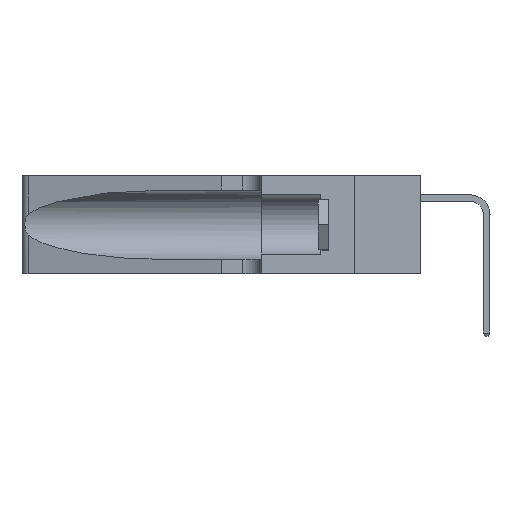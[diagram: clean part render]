
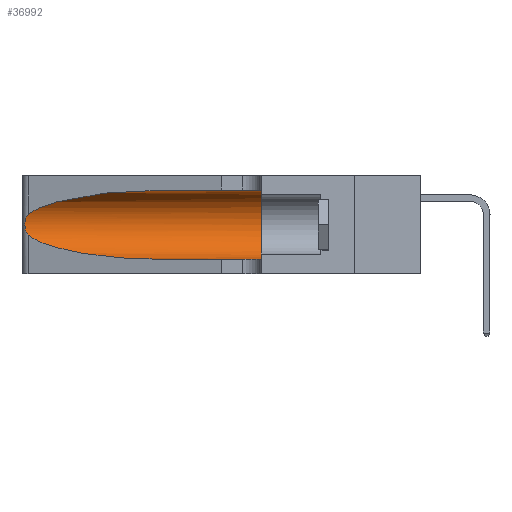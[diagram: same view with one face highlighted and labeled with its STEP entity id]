
A CAD part, left-side view. The second image highlights one B-rep face of the part: STEP entity #36992.
In plain terms, the highlighted cylindrical face has radius 3.308 mm (diameter 6.617 mm), a partial arc.
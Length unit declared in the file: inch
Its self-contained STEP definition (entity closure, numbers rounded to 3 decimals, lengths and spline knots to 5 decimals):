
#2762 = CARTESIAN_POINT ( 'NONE',  ( 0.26018, 1.23835, 0.19895 ) ) ;
#4239 = VECTOR ( 'NONE', #39506, 39.37008 ) ;
#4840 = CARTESIAN_POINT ( 'NONE',  ( 0.1305, 1.61858, 0.05475 ) ) ;
#5601 = CARTESIAN_POINT ( 'NONE',  ( 0.25487, 1.22718, 0.14631 ) ) ;
#6692 = CARTESIAN_POINT ( 'NONE',  ( 0.26075, 1.23896, 0.178 ) ) ;
#6859 = FACE_OUTER_BOUND ( 'NONE', #25412, .T. ) ;
#7450 = CARTESIAN_POINT ( 'NONE',  ( 0.2373, 1.15595, 0.08982 ) ) ;
#9319 = DIRECTION ( 'NONE',  ( 0., -1., 0. ) ) ;
#9712 = CARTESIAN_POINT ( 'NONE',  ( 0.25487, 1.22718, 0.22369 ) ) ;
#10276 = EDGE_CURVE ( 'NONE', #11919, #13698, #40772, .T. ) ;
#10569 = CARTESIAN_POINT ( 'NONE',  ( 0.25856, 1.23593, 0.16098 ) ) ;
#11341 = CARTESIAN_POINT ( 'NONE',  ( 0.1305, 0.35, 0.185 ) ) ;
#11919 = VERTEX_POINT ( 'NONE', #27972 ) ;
#12589 = ORIENTED_EDGE ( 'NONE', *, *, #13298, .T. ) ;
#12993 = CARTESIAN_POINT ( 'NONE',  ( 0.1305, 1.61858, 0.185 ) ) ;
#13034 = CARTESIAN_POINT ( 'NONE',  ( 0.1305, 1.61858, 0.31525 ) ) ;
#13298 = EDGE_CURVE ( 'NONE', #17038, #47004, #18634, .T. ) ;
#13664 = EDGE_CURVE ( 'NONE', #35030, #39182, #22699, .T. ) ;
#13698 = VERTEX_POINT ( 'NONE', #15525 ) ;
#14442 = ORIENTED_EDGE ( 'NONE', *, *, #18307, .T. ) ;
#14448 = CARTESIAN_POINT ( 'NONE',  ( 0.25639, 1.23186, 0.15144 ) ) ;
#15202 = CARTESIAN_POINT ( 'NONE',  ( 0.25487, 1.22718, 0.14631 ) ) ;
#15211 = DIRECTION ( 'NONE',  ( 0., 0., 1. ) ) ;
#15525 = CARTESIAN_POINT ( 'NONE',  ( 0.1305, 0.35, 0.05475 ) ) ;
#16726 = CARTESIAN_POINT ( 'NONE',  ( 0.2373, 1.15595, 0.28018 ) ) ;
#17038 = VERTEX_POINT ( 'NONE', #23335 ) ;
#18133 = CARTESIAN_POINT ( 'NONE',  ( 0.25487, 1.22718, 0.22369 ) ) ;
#18303 = CARTESIAN_POINT ( 'NONE',  ( 0.25487, 1.22718, 0.14631 ) ) ;
#18307 = EDGE_CURVE ( 'NONE', #39182, #13698, #36179, .T. ) ;
#18634 =( BOUNDED_CURVE ( )  B_SPLINE_CURVE ( 3, ( #47461, #20584, #16726, #24452 ),
 .UNSPECIFIED., .F., .F. ) 
 B_SPLINE_CURVE_WITH_KNOTS ( ( 4, 4 ),
 ( 1.5708, 2.84003 ),
 .UNSPECIFIED. ) 
 CURVE ( )  GEOMETRIC_REPRESENTATION_ITEM ( )  RATIONAL_B_SPLINE_CURVE ( ( 1., 0.87, 0.87, 1. ) ) 
 REPRESENTATION_ITEM ( '' )  );
#20584 = CARTESIAN_POINT ( 'NONE',  ( 0.18966, 0.96281, 0.31525 ) ) ;
#20757 = AXIS2_PLACEMENT_3D ( 'NONE', #11341, #38213, #15211 ) ;
#21016 = ORIENTED_EDGE ( 'NONE', *, *, #13664, .T. ) ;
#21658 = VECTOR ( 'NONE', #9319, 39.37008 ) ;
#22022 = CARTESIAN_POINT ( 'NONE',  ( 0.25639, 1.23184, 0.21858 ) ) ;
#22699 =( BOUNDED_CURVE ( )  B_SPLINE_CURVE ( 3, ( #15202, #7450, #49630, #42070 ),
 .UNSPECIFIED., .F., .F. ) 
 B_SPLINE_CURVE_WITH_KNOTS ( ( 4, 4 ),
 ( 3.44316, 4.71239 ),
 .UNSPECIFIED. ) 
 CURVE ( )  GEOMETRIC_REPRESENTATION_ITEM ( )  RATIONAL_B_SPLINE_CURVE ( ( 1., 0.87, 0.87, 1. ) ) 
 REPRESENTATION_ITEM ( '' )  );
#22843 = ORIENTED_EDGE ( 'NONE', *, *, #26994, .T. ) ;
#23335 = CARTESIAN_POINT ( 'NONE',  ( 0.1305, 0.72297, 0.31525 ) ) ;
#23591 = AXIS2_PLACEMENT_3D ( 'NONE', #12993, #47426, #39866 ) ;
#24452 = CARTESIAN_POINT ( 'NONE',  ( 0.25487, 1.22718, 0.22369 ) ) ;
#25412 = EDGE_LOOP ( 'NONE', ( #12589, #22843, #21016, #14442, #38484, #48712 ) ) ;
#25880 = CARTESIAN_POINT ( 'NONE',  ( 0.25854, 1.2359, 0.20912 ) ) ;
#26994 = EDGE_CURVE ( 'NONE', #47004, #35030, #39233, .T. ) ;
#27972 = CARTESIAN_POINT ( 'NONE',  ( 0.1305, 0.35, 0.31525 ) ) ;
#29728 = CARTESIAN_POINT ( 'NONE',  ( 0.26075, 1.23896, 0.19203 ) ) ;
#33606 = CARTESIAN_POINT ( 'NONE',  ( 0.26017, 1.23833, 0.17102 ) ) ;
#35030 = VERTEX_POINT ( 'NONE', #5601 ) ;
#35512 = LINE ( 'NONE', #13034, #21658 ) ;
#36179 = LINE ( 'NONE', #4840, #4239 ) ;
#36338 = CYLINDRICAL_SURFACE ( 'NONE', #23591, 0.13025 ) ;
#36992 = ADVANCED_FACE ( 'NONE', ( #6859 ), #36338, .F. ) ;
#37299 = CARTESIAN_POINT ( 'NONE',  ( 0.25555, 1.22994, 0.2215 ) ) ;
#37469 = CARTESIAN_POINT ( 'NONE',  ( 0.25789, 1.23486, 0.15765 ) ) ;
#38213 = DIRECTION ( 'NONE',  ( 0., 1., 0. ) ) ;
#38484 = ORIENTED_EDGE ( 'NONE', *, *, #10276, .F. ) ;
#39182 = VERTEX_POINT ( 'NONE', #48930 ) ;
#39233 = B_SPLINE_CURVE_WITH_KNOTS ( 'NONE', 3,
 ( #18133, #37299, #22022, #48893, #25880, #2762, #29728, #6692, #33606, #10569, #37469, #14448, #41334, #18303 ),
 .UNSPECIFIED., .F., .F.,
 ( 4, 2, 2, 2, 2, 2, 4 ),
 ( 0., 0.00027, 0.00053, 0.00107, 0.0016, 0.00187, 0.00214 ),
 .UNSPECIFIED. ) ;
#39506 = DIRECTION ( 'NONE',  ( 0., -1., 0. ) ) ;
#39866 = DIRECTION ( 'NONE',  ( 0., 0., -1. ) ) ;
#40772 = CIRCLE ( 'NONE', #20757, 0.13025 ) ;
#41334 = CARTESIAN_POINT ( 'NONE',  ( 0.25555, 1.22993, 0.14849 ) ) ;
#42070 = CARTESIAN_POINT ( 'NONE',  ( 0.1305, 0.72297, 0.05475 ) ) ;
#47004 = VERTEX_POINT ( 'NONE', #9712 ) ;
#47426 = DIRECTION ( 'NONE',  ( 0., -1., 0. ) ) ;
#47461 = CARTESIAN_POINT ( 'NONE',  ( 0.1305, 0.72297, 0.31525 ) ) ;
#47573 = EDGE_CURVE ( 'NONE', #17038, #11919, #35512, .T. ) ;
#48712 = ORIENTED_EDGE ( 'NONE', *, *, #47573, .F. ) ;
#48893 = CARTESIAN_POINT ( 'NONE',  ( 0.25787, 1.23484, 0.2124 ) ) ;
#48930 = CARTESIAN_POINT ( 'NONE',  ( 0.1305, 0.72297, 0.05475 ) ) ;
#49630 = CARTESIAN_POINT ( 'NONE',  ( 0.18966, 0.96281, 0.05475 ) ) ;
